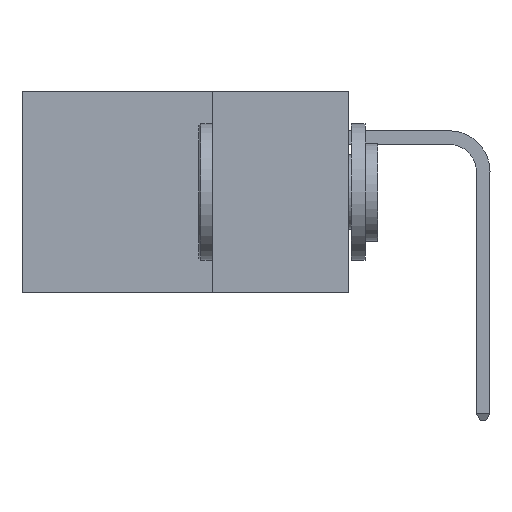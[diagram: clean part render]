
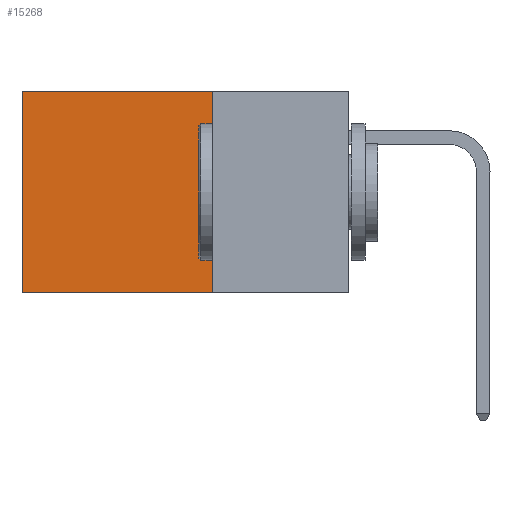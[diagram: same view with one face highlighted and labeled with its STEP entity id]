
A CAD part, left-side view. The second image highlights one B-rep face of the part: STEP entity #15268.
In plain terms, the highlighted planar face has unit normal (-1, 0, 0).
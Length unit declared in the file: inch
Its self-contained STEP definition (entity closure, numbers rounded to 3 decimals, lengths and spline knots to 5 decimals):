
#150 = VERTEX_POINT ( 'NONE', #26059 ) ;
#898 = CARTESIAN_POINT ( 'NONE',  ( 0.2875, 0.25, 0. ) ) ;
#2267 = CARTESIAN_POINT ( 'NONE',  ( 0.2875, 0.25, -0.37 ) ) ;
#2551 = VECTOR ( 'NONE', #21208, 39.37008 ) ;
#3338 = FACE_OUTER_BOUND ( 'NONE', #5437, .T. ) ;
#5112 = CARTESIAN_POINT ( 'NONE',  ( 0.2875, 0.6, -0.37 ) ) ;
#5437 = EDGE_LOOP ( 'NONE', ( #11849, #21703, #24763, #14360 ) ) ;
#5820 = EDGE_CURVE ( 'NONE', #150, #9409, #20351, .T. ) ;
#6511 = DIRECTION ( 'NONE',  ( 0., 0., -1. ) ) ;
#7648 = DIRECTION ( 'NONE',  ( 0., 0., -1. ) ) ;
#8950 = VERTEX_POINT ( 'NONE', #19752 ) ;
#9409 = VERTEX_POINT ( 'NONE', #5112 ) ;
#11116 = VECTOR ( 'NONE', #15719, 39.37008 ) ;
#11849 = ORIENTED_EDGE ( 'NONE', *, *, #33701, .T. ) ;
#12900 = CARTESIAN_POINT ( 'NONE',  ( 0.2875, 0.25, 0. ) ) ;
#13746 = VECTOR ( 'NONE', #7648, 39.37008 ) ;
#14360 = ORIENTED_EDGE ( 'NONE', *, *, #33336, .T. ) ;
#15268 = ADVANCED_FACE ( 'NONE', ( #3338 ), #20392, .F. ) ;
#15593 = CARTESIAN_POINT ( 'NONE',  ( 0.2875, 0.25, 0. ) ) ;
#15719 = DIRECTION ( 'NONE',  ( 0., 1., 0. ) ) ;
#16509 = VERTEX_POINT ( 'NONE', #24554 ) ;
#19752 = CARTESIAN_POINT ( 'NONE',  ( 0.2875, 0.25, 0. ) ) ;
#20351 = LINE ( 'NONE', #2267, #32552 ) ;
#20392 = PLANE ( 'NONE',  #32400 ) ;
#21208 = DIRECTION ( 'NONE',  ( 0., 0., -1. ) ) ;
#21703 = ORIENTED_EDGE ( 'NONE', *, *, #5820, .F. ) ;
#22290 = EDGE_CURVE ( 'NONE', #8950, #150, #24771, .T. ) ;
#23188 = DIRECTION ( 'NONE',  ( 1., 0., 0. ) ) ;
#24542 = DIRECTION ( 'NONE',  ( 0., 1., 0. ) ) ;
#24554 = CARTESIAN_POINT ( 'NONE',  ( 0.2875, 0.6, 0. ) ) ;
#24763 = ORIENTED_EDGE ( 'NONE', *, *, #22290, .F. ) ;
#24771 = LINE ( 'NONE', #15593, #2551 ) ;
#26059 = CARTESIAN_POINT ( 'NONE',  ( 0.2875, 0.25, -0.37 ) ) ;
#28564 = LINE ( 'NONE', #29990, #13746 ) ;
#29990 = CARTESIAN_POINT ( 'NONE',  ( 0.2875, 0.6, 0. ) ) ;
#32400 = AXIS2_PLACEMENT_3D ( 'NONE', #898, #23188, #6511 ) ;
#32552 = VECTOR ( 'NONE', #24542, 39.37008 ) ;
#33336 = EDGE_CURVE ( 'NONE', #8950, #16509, #34265, .T. ) ;
#33701 = EDGE_CURVE ( 'NONE', #16509, #9409, #28564, .T. ) ;
#34265 = LINE ( 'NONE', #12900, #11116 ) ;
